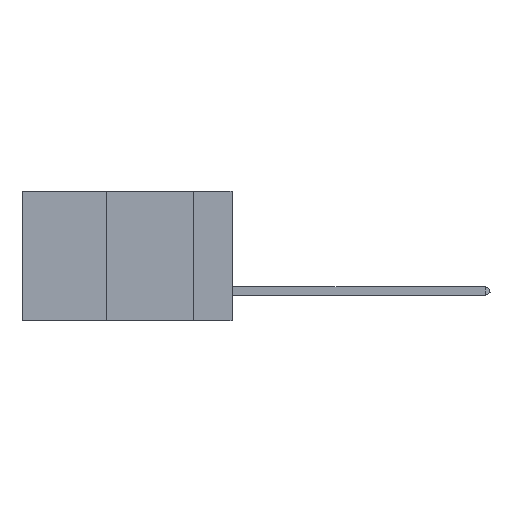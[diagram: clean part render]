
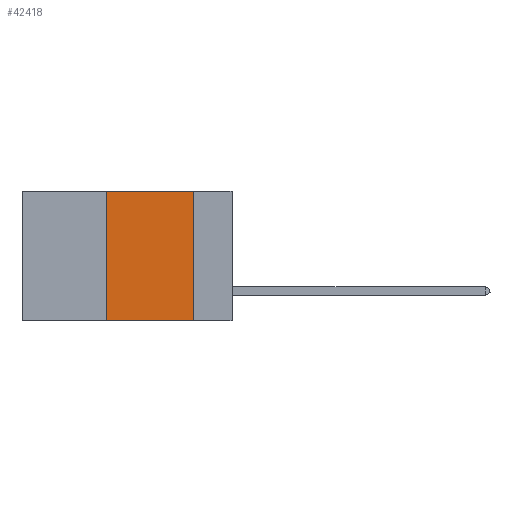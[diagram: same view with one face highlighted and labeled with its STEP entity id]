
A CAD part, left-side view. The second image highlights one B-rep face of the part: STEP entity #42418.
In plain terms, the highlighted planar face has unit normal (-1, 0, 0).
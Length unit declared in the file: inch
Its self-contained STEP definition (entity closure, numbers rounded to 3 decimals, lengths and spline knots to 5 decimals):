
#241 = LINE ( 'NONE', #39085, #46236 ) ;
#283 = DIRECTION ( 'NONE',  ( 0., 0., -1. ) ) ;
#2019 = ORIENTED_EDGE ( 'NONE', *, *, #11526, .F. ) ;
#3900 = LINE ( 'NONE', #40445, #14976 ) ;
#4073 = PLANE ( 'NONE',  #46038 ) ;
#4596 = CARTESIAN_POINT ( 'NONE',  ( 0., 0.6, 0. ) ) ;
#7335 = DIRECTION ( 'NONE',  ( 0., 0., -1. ) ) ;
#10722 = CARTESIAN_POINT ( 'NONE',  ( 0., 0.36, -0.37 ) ) ;
#11526 = EDGE_CURVE ( 'NONE', #16337, #16482, #3900, .T. ) ;
#13340 = EDGE_CURVE ( 'NONE', #16337, #14539, #241, .T. ) ;
#14539 = VERTEX_POINT ( 'NONE', #17526 ) ;
#14976 = VECTOR ( 'NONE', #36379, 39.37008 ) ;
#16337 = VERTEX_POINT ( 'NONE', #10722 ) ;
#16482 = VERTEX_POINT ( 'NONE', #26085 ) ;
#17526 = CARTESIAN_POINT ( 'NONE',  ( 0., 0.11, -0.37 ) ) ;
#18568 = EDGE_CURVE ( 'NONE', #44581, #14539, #40421, .T. ) ;
#18866 = CARTESIAN_POINT ( 'NONE',  ( 0., 0.11, 0. ) ) ;
#20216 = ORIENTED_EDGE ( 'NONE', *, *, #18568, .F. ) ;
#21906 = ORIENTED_EDGE ( 'NONE', *, *, #13340, .T. ) ;
#26085 = CARTESIAN_POINT ( 'NONE',  ( 0., 0.36, 0. ) ) ;
#26334 = CARTESIAN_POINT ( 'NONE',  ( 0., 0.6, 0. ) ) ;
#31810 = LINE ( 'NONE', #4596, #34170 ) ;
#32192 = FACE_OUTER_BOUND ( 'NONE', #43318, .T. ) ;
#32734 = DIRECTION ( 'NONE',  ( 0., -1., 0. ) ) ;
#33826 = DIRECTION ( 'NONE',  ( 1., 0., 0. ) ) ;
#34170 = VECTOR ( 'NONE', #34519, 39.37008 ) ;
#34519 = DIRECTION ( 'NONE',  ( 0., -1., 0. ) ) ;
#35761 = VECTOR ( 'NONE', #283, 39.37008 ) ;
#36379 = DIRECTION ( 'NONE',  ( 0., 0., 1. ) ) ;
#39085 = CARTESIAN_POINT ( 'NONE',  ( 0., 0.6, -0.37 ) ) ;
#40421 = LINE ( 'NONE', #44862, #35761 ) ;
#40445 = CARTESIAN_POINT ( 'NONE',  ( 0., 0.36, 0. ) ) ;
#42418 = ADVANCED_FACE ( 'NONE', ( #32192 ), #4073, .F. ) ;
#43318 = EDGE_LOOP ( 'NONE', ( #20216, #48178, #2019, #21906 ) ) ;
#44581 = VERTEX_POINT ( 'NONE', #18866 ) ;
#44862 = CARTESIAN_POINT ( 'NONE',  ( 0., 0.11, 0. ) ) ;
#46038 = AXIS2_PLACEMENT_3D ( 'NONE', #26334, #33826, #7335 ) ;
#46236 = VECTOR ( 'NONE', #32734, 39.37008 ) ;
#46942 = EDGE_CURVE ( 'NONE', #16482, #44581, #31810, .T. ) ;
#48178 = ORIENTED_EDGE ( 'NONE', *, *, #46942, .F. ) ;
